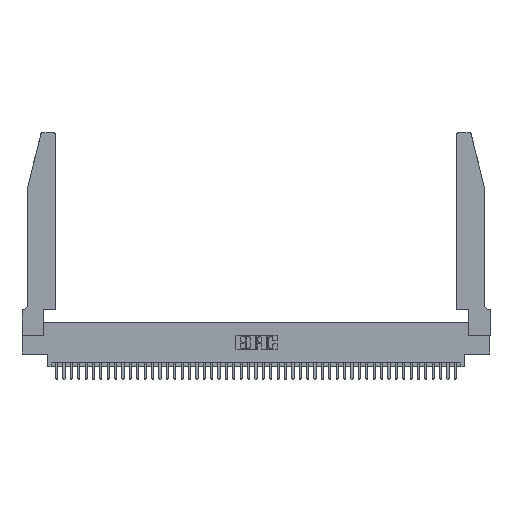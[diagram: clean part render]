
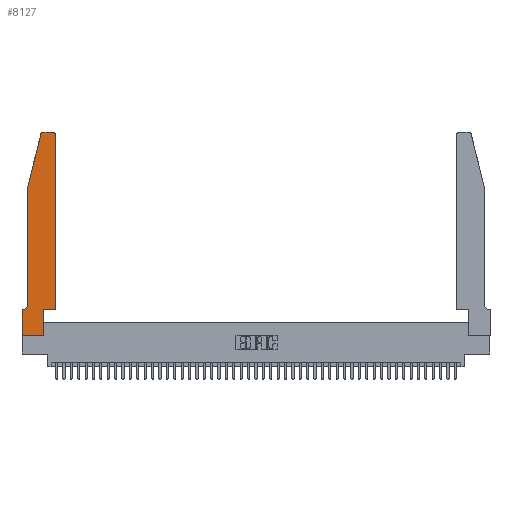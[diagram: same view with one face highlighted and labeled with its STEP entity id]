
A CAD part, top view. The second image highlights one B-rep face of the part: STEP entity #8127.
In plain terms, the highlighted planar face has unit normal (0, 0, 1).
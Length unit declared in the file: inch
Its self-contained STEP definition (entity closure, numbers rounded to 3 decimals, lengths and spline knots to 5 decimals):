
#14 = VERTEX_POINT ( 'NONE', #40382 ) ;
#474 = DIRECTION ( 'NONE',  ( 1., 0., 0. ) ) ;
#732 = CARTESIAN_POINT ( 'NONE',  ( 0., 0., 0.37 ) ) ;
#1332 = VECTOR ( 'NONE', #474, 39.37008 ) ;
#1858 = VERTEX_POINT ( 'NONE', #30140 ) ;
#2158 = CARTESIAN_POINT ( 'NONE',  ( 0.2605, 2.75, 0.37 ) ) ;
#2231 = EDGE_CURVE ( 'NONE', #39103, #13793, #16124, .T. ) ;
#2715 = CARTESIAN_POINT ( 'NONE',  ( 0.0755, 0.42, 0.37 ) ) ;
#2955 = EDGE_CURVE ( 'NONE', #13793, #7406, #14942, .T. ) ;
#3830 = VERTEX_POINT ( 'NONE', #38061 ) ;
#4027 = ORIENTED_EDGE ( 'NONE', *, *, #8656, .T. ) ;
#4074 = DIRECTION ( 'NONE',  ( 1., 0., 0. ) ) ;
#4562 = ORIENTED_EDGE ( 'NONE', *, *, #2955, .T. ) ;
#5051 = LINE ( 'NONE', #28851, #1332 ) ;
#5804 = ORIENTED_EDGE ( 'NONE', *, *, #26008, .T. ) ;
#7069 = ORIENTED_EDGE ( 'NONE', *, *, #16389, .T. ) ;
#7406 = VERTEX_POINT ( 'NONE', #26191 ) ;
#8127 = ADVANCED_FACE ( 'NONE', ( #38693 ), #36780, .T. ) ;
#8344 = DIRECTION ( 'NONE',  ( 0., 1., 0. ) ) ;
#8588 = EDGE_CURVE ( 'NONE', #41822, #14, #5051, .T. ) ;
#8656 = EDGE_CURVE ( 'NONE', #39730, #41822, #26901, .T. ) ;
#8722 = VECTOR ( 'NONE', #29129, 39.37008 ) ;
#8995 = EDGE_CURVE ( 'NONE', #7406, #1858, #18973, .T. ) ;
#9552 = CARTESIAN_POINT ( 'NONE',  ( 0.0055, 0.42, 0.37 ) ) ;
#9836 = CIRCLE ( 'NONE', #19245, 0.03 ) ;
#10191 = AXIS2_PLACEMENT_3D ( 'NONE', #24225, #41700, #20158 ) ;
#10282 = CARTESIAN_POINT ( 'NONE',  ( 0., 0.35, 0.37 ) ) ;
#10490 = VERTEX_POINT ( 'NONE', #32275 ) ;
#11226 = VECTOR ( 'NONE', #42915, 39.37008 ) ;
#11831 = LINE ( 'NONE', #28658, #11226 ) ;
#11986 = CIRCLE ( 'NONE', #13030, 0.07 ) ;
#13030 = AXIS2_PLACEMENT_3D ( 'NONE', #9552, #13156, #20029 ) ;
#13156 = DIRECTION ( 'NONE',  ( 0., 0., -1. ) ) ;
#13793 = VERTEX_POINT ( 'NONE', #36844 ) ;
#14168 = DIRECTION ( 'NONE',  ( 0., 1., 0. ) ) ;
#14226 = ORIENTED_EDGE ( 'NONE', *, *, #15713, .T. ) ;
#14290 = VECTOR ( 'NONE', #8344, 39.37008 ) ;
#14745 = VERTEX_POINT ( 'NONE', #2715 ) ;
#14942 = CIRCLE ( 'NONE', #10191, 0.03 ) ;
#15713 = EDGE_CURVE ( 'NONE', #10490, #39103, #9836, .T. ) ;
#15895 = DIRECTION ( 'NONE',  ( 0., -1., 0. ) ) ;
#16124 = LINE ( 'NONE', #2158, #42495 ) ;
#16389 = EDGE_CURVE ( 'NONE', #16442, #39730, #38428, .T. ) ;
#16442 = VERTEX_POINT ( 'NONE', #39765 ) ;
#16705 = EDGE_CURVE ( 'NONE', #1858, #14745, #45121, .T. ) ;
#17249 = VECTOR ( 'NONE', #23095, 39.37008 ) ;
#17270 = VECTOR ( 'NONE', #31347, 39.37008 ) ;
#17485 = ORIENTED_EDGE ( 'NONE', *, *, #16705, .T. ) ;
#18273 = EDGE_LOOP ( 'NONE', ( #22022, #4562, #39085, #17485, #29408, #7069, #4027, #23112, #20534, #5804, #29326, #14226 ) ) ;
#18545 = DIRECTION ( 'NONE',  ( 0., 0., 1. ) ) ;
#18973 = LINE ( 'NONE', #44622, #17249 ) ;
#19034 = CARTESIAN_POINT ( 'NONE',  ( 0.4205, 2.75, 0.37 ) ) ;
#19245 = AXIS2_PLACEMENT_3D ( 'NONE', #43118, #39503, #4074 ) ;
#20029 = DIRECTION ( 'NONE',  ( -1., 0., 0. ) ) ;
#20158 = DIRECTION ( 'NONE',  ( 1., 0., 0. ) ) ;
#20534 = ORIENTED_EDGE ( 'NONE', *, *, #29566, .T. ) ;
#21932 = VECTOR ( 'NONE', #14168, 39.37008 ) ;
#22022 = ORIENTED_EDGE ( 'NONE', *, *, #2231, .T. ) ;
#23095 = DIRECTION ( 'NONE',  ( -0.239, -0.971, 0. ) ) ;
#23112 = ORIENTED_EDGE ( 'NONE', *, *, #8588, .T. ) ;
#23750 = VECTOR ( 'NONE', #15895, 39.37008 ) ;
#24225 = CARTESIAN_POINT ( 'NONE',  ( 0.284, 2.72, 0.37 ) ) ;
#25136 = CARTESIAN_POINT ( 'NONE',  ( 0.0755, 0.35, 0.37 ) ) ;
#25306 = DIRECTION ( 'NONE',  ( 1., 0., 0. ) ) ;
#25562 = CARTESIAN_POINT ( 'NONE',  ( 0., 0., 0.37 ) ) ;
#26008 = EDGE_CURVE ( 'NONE', #35649, #3830, #11831, .T. ) ;
#26078 = LINE ( 'NONE', #29833, #14290 ) ;
#26191 = CARTESIAN_POINT ( 'NONE',  ( 0.25487, 2.72718, 0.37 ) ) ;
#26901 = LINE ( 'NONE', #25562, #17270 ) ;
#28658 = CARTESIAN_POINT ( 'NONE',  ( 0.4505, 0.35, 0.37 ) ) ;
#28851 = CARTESIAN_POINT ( 'NONE',  ( 0., 0., 0.37 ) ) ;
#29129 = DIRECTION ( 'NONE',  ( -1., 0., 0. ) ) ;
#29326 = ORIENTED_EDGE ( 'NONE', *, *, #31492, .T. ) ;
#29408 = ORIENTED_EDGE ( 'NONE', *, *, #33733, .T. ) ;
#29450 = CARTESIAN_POINT ( 'NONE',  ( 0., 0.35, 0.37 ) ) ;
#29566 = EDGE_CURVE ( 'NONE', #14, #35649, #26078, .T. ) ;
#29833 = CARTESIAN_POINT ( 'NONE',  ( 0.2865, 0.35, 0.37 ) ) ;
#30140 = CARTESIAN_POINT ( 'NONE',  ( 0.0755, 2., 0.37 ) ) ;
#30458 = LINE ( 'NONE', #39261, #21932 ) ;
#30526 = CARTESIAN_POINT ( 'NONE',  ( 0.0755, 2., 0.37 ) ) ;
#30672 = DIRECTION ( 'NONE',  ( -1., 0., 0. ) ) ;
#31225 = CARTESIAN_POINT ( 'NONE',  ( 0.2865, 0.35, 0.37 ) ) ;
#31347 = DIRECTION ( 'NONE',  ( 0., -1., 0. ) ) ;
#31492 = EDGE_CURVE ( 'NONE', #3830, #10490, #30458, .T. ) ;
#32195 = AXIS2_PLACEMENT_3D ( 'NONE', #29450, #18545, #25306 ) ;
#32275 = CARTESIAN_POINT ( 'NONE',  ( 0.4505, 2.72, 0.37 ) ) ;
#33733 = EDGE_CURVE ( 'NONE', #14745, #16442, #11986, .T. ) ;
#35649 = VERTEX_POINT ( 'NONE', #31225 ) ;
#36780 = PLANE ( 'NONE',  #32195 ) ;
#36844 = CARTESIAN_POINT ( 'NONE',  ( 0.284, 2.75, 0.37 ) ) ;
#38061 = CARTESIAN_POINT ( 'NONE',  ( 0.4505, 0.35, 0.37 ) ) ;
#38428 = LINE ( 'NONE', #25136, #8722 ) ;
#38693 = FACE_OUTER_BOUND ( 'NONE', #18273, .T. ) ;
#39085 = ORIENTED_EDGE ( 'NONE', *, *, #8995, .T. ) ;
#39103 = VERTEX_POINT ( 'NONE', #19034 ) ;
#39261 = CARTESIAN_POINT ( 'NONE',  ( 0.4505, 0.35, 0.37 ) ) ;
#39503 = DIRECTION ( 'NONE',  ( 0., 0., 1. ) ) ;
#39730 = VERTEX_POINT ( 'NONE', #10282 ) ;
#39765 = CARTESIAN_POINT ( 'NONE',  ( 0.0055, 0.35, 0.37 ) ) ;
#40382 = CARTESIAN_POINT ( 'NONE',  ( 0.2865, 0., 0.37 ) ) ;
#41700 = DIRECTION ( 'NONE',  ( 0., 0., 1. ) ) ;
#41822 = VERTEX_POINT ( 'NONE', #732 ) ;
#42495 = VECTOR ( 'NONE', #30672, 39.37008 ) ;
#42915 = DIRECTION ( 'NONE',  ( 1., 0., 0. ) ) ;
#43118 = CARTESIAN_POINT ( 'NONE',  ( 0.4205, 2.72, 0.37 ) ) ;
#44622 = CARTESIAN_POINT ( 'NONE',  ( 0.0755, 2., 0.37 ) ) ;
#45121 = LINE ( 'NONE', #30526, #23750 ) ;
